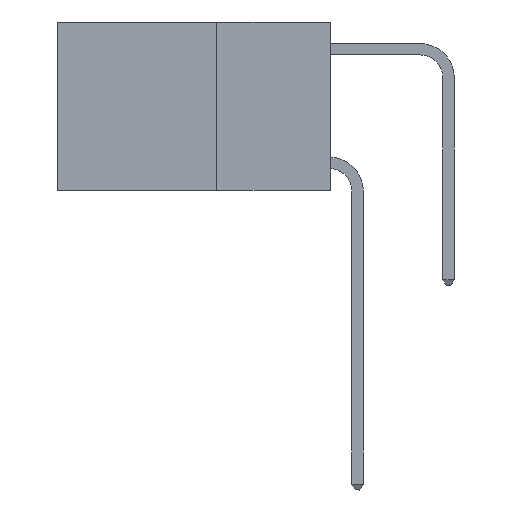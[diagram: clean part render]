
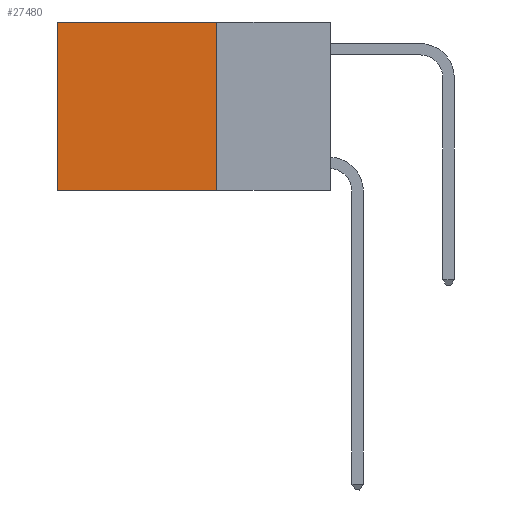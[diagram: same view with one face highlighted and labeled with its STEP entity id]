
A CAD part, left-side view. The second image highlights one B-rep face of the part: STEP entity #27480.
In plain terms, the highlighted planar face has unit normal (-1, 0, 0).
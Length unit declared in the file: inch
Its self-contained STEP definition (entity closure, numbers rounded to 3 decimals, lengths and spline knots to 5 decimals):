
#326 = VECTOR ( 'NONE', #18390, 39.37008 ) ;
#1300 = VECTOR ( 'NONE', #22451, 39.37008 ) ;
#1630 = ORIENTED_EDGE ( 'NONE', *, *, #11018, .F. ) ;
#1969 = CARTESIAN_POINT ( 'NONE',  ( 0.2625, 0.25, -0.37 ) ) ;
#2168 = EDGE_LOOP ( 'NONE', ( #22013, #1630, #20409, #3200 ) ) ;
#2305 = CARTESIAN_POINT ( 'NONE',  ( 0.2625, 0.25, 0. ) ) ;
#3200 = ORIENTED_EDGE ( 'NONE', *, *, #19718, .T. ) ;
#3872 = FACE_OUTER_BOUND ( 'NONE', #2168, .T. ) ;
#5018 = VECTOR ( 'NONE', #15364, 39.37008 ) ;
#5056 = LINE ( 'NONE', #18027, #1300 ) ;
#6451 = PLANE ( 'NONE',  #22068 ) ;
#10412 = DIRECTION ( 'NONE',  ( 1., 0., 0. ) ) ;
#10875 = LINE ( 'NONE', #16779, #25270 ) ;
#11018 = EDGE_CURVE ( 'NONE', #18010, #26667, #10875, .T. ) ;
#13532 = EDGE_CURVE ( 'NONE', #24948, #26667, #27539, .T. ) ;
#14189 = EDGE_CURVE ( 'NONE', #26409, #18010, #16487, .T. ) ;
#14201 = CARTESIAN_POINT ( 'NONE',  ( 0.2625, 0.6, -0.37 ) ) ;
#15364 = DIRECTION ( 'NONE',  ( 0., 0., -1. ) ) ;
#16487 = LINE ( 'NONE', #2305, #5018 ) ;
#16779 = CARTESIAN_POINT ( 'NONE',  ( 0.2625, 0.25, -0.37 ) ) ;
#18010 = VERTEX_POINT ( 'NONE', #1969 ) ;
#18027 = CARTESIAN_POINT ( 'NONE',  ( 0.2625, 0.25, 0. ) ) ;
#18390 = DIRECTION ( 'NONE',  ( 0., 0., -1. ) ) ;
#18903 = CARTESIAN_POINT ( 'NONE',  ( 0.2625, 0.6, 0. ) ) ;
#19718 = EDGE_CURVE ( 'NONE', #26409, #24948, #5056, .T. ) ;
#20409 = ORIENTED_EDGE ( 'NONE', *, *, #14189, .F. ) ;
#20611 = CARTESIAN_POINT ( 'NONE',  ( 0.2625, 0.6, 0. ) ) ;
#21380 = CARTESIAN_POINT ( 'NONE',  ( 0.2625, 0.25, 0. ) ) ;
#21433 = DIRECTION ( 'NONE',  ( 0., 1., 0. ) ) ;
#21745 = CARTESIAN_POINT ( 'NONE',  ( 0.2625, 0.25, 0. ) ) ;
#22013 = ORIENTED_EDGE ( 'NONE', *, *, #13532, .T. ) ;
#22068 = AXIS2_PLACEMENT_3D ( 'NONE', #21380, #10412, #25501 ) ;
#22451 = DIRECTION ( 'NONE',  ( 0., 1., 0. ) ) ;
#24948 = VERTEX_POINT ( 'NONE', #18903 ) ;
#25270 = VECTOR ( 'NONE', #21433, 39.37008 ) ;
#25501 = DIRECTION ( 'NONE',  ( 0., 0., -1. ) ) ;
#26409 = VERTEX_POINT ( 'NONE', #21745 ) ;
#26667 = VERTEX_POINT ( 'NONE', #14201 ) ;
#27480 = ADVANCED_FACE ( 'NONE', ( #3872 ), #6451, .F. ) ;
#27539 = LINE ( 'NONE', #20611, #326 ) ;
